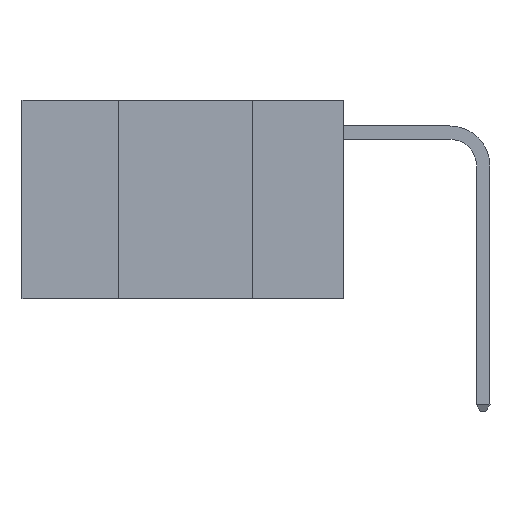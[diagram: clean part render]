
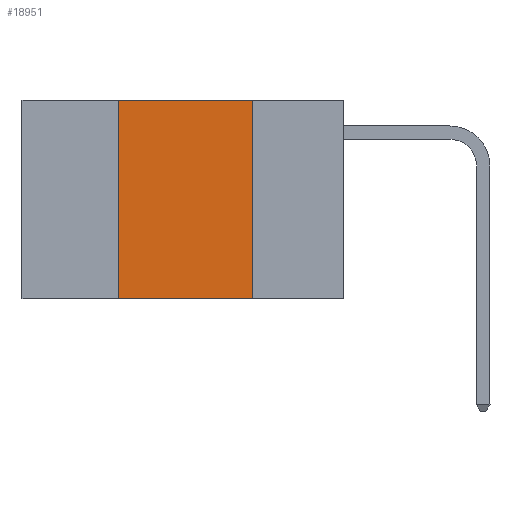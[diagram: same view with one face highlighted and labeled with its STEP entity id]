
A CAD part, left-side view. The second image highlights one B-rep face of the part: STEP entity #18951.
In plain terms, the highlighted planar face has unit normal (-1, 0, 0).
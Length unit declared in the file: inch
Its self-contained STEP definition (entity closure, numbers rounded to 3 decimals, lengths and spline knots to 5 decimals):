
#132 = AXIS2_PLACEMENT_3D ( 'NONE', #18697, #10295, #1144 ) ;
#306 = VECTOR ( 'NONE', #3462, 39.37008 ) ;
#706 = DIRECTION ( 'NONE',  ( 0., -1., 0. ) ) ;
#792 = CARTESIAN_POINT ( 'NONE',  ( 0., 0.6, 0. ) ) ;
#1144 = DIRECTION ( 'NONE',  ( 0., 0., -1. ) ) ;
#1701 = VERTEX_POINT ( 'NONE', #7183 ) ;
#2346 = DIRECTION ( 'NONE',  ( 0., -1., 0. ) ) ;
#2436 = CARTESIAN_POINT ( 'NONE',  ( 0., 0.6, -0.37 ) ) ;
#3152 = VERTEX_POINT ( 'NONE', #15735 ) ;
#3462 = DIRECTION ( 'NONE',  ( 0., 0., 1. ) ) ;
#4388 = ORIENTED_EDGE ( 'NONE', *, *, #4501, .F. ) ;
#4423 = LINE ( 'NONE', #15375, #306 ) ;
#4501 = EDGE_CURVE ( 'NONE', #3152, #9976, #6328, .T. ) ;
#4596 = ORIENTED_EDGE ( 'NONE', *, *, #10427, .F. ) ;
#6328 = LINE ( 'NONE', #792, #17371 ) ;
#6604 = FACE_OUTER_BOUND ( 'NONE', #18554, .T. ) ;
#6929 = DIRECTION ( 'NONE',  ( 0., 0., -1. ) ) ;
#7183 = CARTESIAN_POINT ( 'NONE',  ( 0., 0.42, -0.37 ) ) ;
#7913 = EDGE_CURVE ( 'NONE', #1701, #11607, #16211, .T. ) ;
#8385 = CARTESIAN_POINT ( 'NONE',  ( 0., 0.17, 0. ) ) ;
#8579 = VECTOR ( 'NONE', #2346, 39.37008 ) ;
#8956 = ORIENTED_EDGE ( 'NONE', *, *, #12388, .F. ) ;
#9287 = CARTESIAN_POINT ( 'NONE',  ( 0., 0.17, -0.37 ) ) ;
#9976 = VERTEX_POINT ( 'NONE', #14771 ) ;
#10295 = DIRECTION ( 'NONE',  ( 1., 0., 0. ) ) ;
#10427 = EDGE_CURVE ( 'NONE', #9976, #11607, #14997, .T. ) ;
#11171 = VECTOR ( 'NONE', #6929, 39.37008 ) ;
#11607 = VERTEX_POINT ( 'NONE', #9287 ) ;
#12388 = EDGE_CURVE ( 'NONE', #1701, #3152, #4423, .T. ) ;
#14650 = PLANE ( 'NONE',  #132 ) ;
#14771 = CARTESIAN_POINT ( 'NONE',  ( 0., 0.17, 0. ) ) ;
#14997 = LINE ( 'NONE', #8385, #11171 ) ;
#15375 = CARTESIAN_POINT ( 'NONE',  ( 0., 0.42, 0. ) ) ;
#15435 = ORIENTED_EDGE ( 'NONE', *, *, #7913, .T. ) ;
#15735 = CARTESIAN_POINT ( 'NONE',  ( 0., 0.42, 0. ) ) ;
#16211 = LINE ( 'NONE', #2436, #8579 ) ;
#17371 = VECTOR ( 'NONE', #706, 39.37008 ) ;
#18554 = EDGE_LOOP ( 'NONE', ( #4596, #4388, #8956, #15435 ) ) ;
#18697 = CARTESIAN_POINT ( 'NONE',  ( 0., 0.6, 0. ) ) ;
#18951 = ADVANCED_FACE ( 'NONE', ( #6604 ), #14650, .F. ) ;
